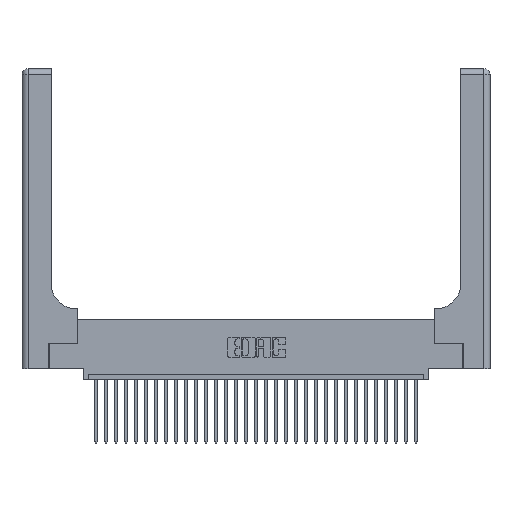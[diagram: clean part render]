
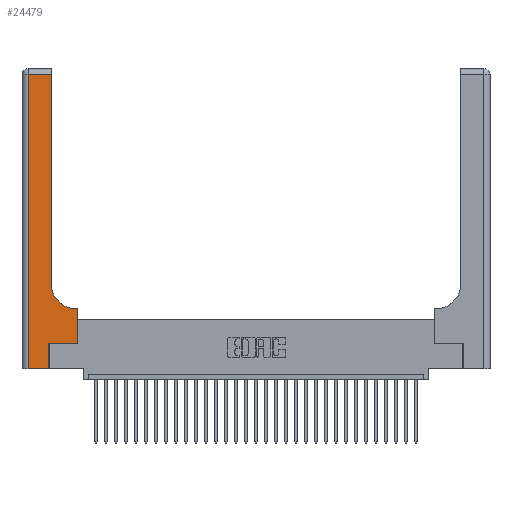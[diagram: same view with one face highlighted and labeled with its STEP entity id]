
A CAD part, top view. The second image highlights one B-rep face of the part: STEP entity #24479.
In plain terms, the highlighted planar face has unit normal (0, 0, 1).
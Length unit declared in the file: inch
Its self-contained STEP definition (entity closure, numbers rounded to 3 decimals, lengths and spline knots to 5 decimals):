
#134 = DIRECTION ( 'NONE',  ( 1., 0., 0. ) ) ;
#626 = VERTEX_POINT ( 'NONE', #4898 ) ;
#785 = DIRECTION ( 'NONE',  ( -1., 0., 0. ) ) ;
#903 = CARTESIAN_POINT ( 'NONE',  ( 0.2915, 0.85, 0.37 ) ) ;
#919 = CARTESIAN_POINT ( 'NONE',  ( 0.06, 3., 0.37 ) ) ;
#1185 = ORIENTED_EDGE ( 'NONE', *, *, #11596, .T. ) ;
#2694 = VERTEX_POINT ( 'NONE', #7220 ) ;
#2824 = VECTOR ( 'NONE', #3640, 39.37008 ) ;
#3193 = AXIS2_PLACEMENT_3D ( 'NONE', #12048, #14713, #22135 ) ;
#3640 = DIRECTION ( 'NONE',  ( 1., 0., 0. ) ) ;
#4898 = CARTESIAN_POINT ( 'NONE',  ( 0.5415, 0.6, 0.37 ) ) ;
#5334 = VECTOR ( 'NONE', #9507, 39.37008 ) ;
#6000 = EDGE_CURVE ( 'NONE', #26856, #626, #19930, .T. ) ;
#6341 = AXIS2_PLACEMENT_3D ( 'NONE', #24748, #12202, #134 ) ;
#7001 = EDGE_CURVE ( 'NONE', #15979, #7440, #29342, .T. ) ;
#7220 = CARTESIAN_POINT ( 'NONE',  ( 0.06, 2.94, 0.37 ) ) ;
#7440 = VERTEX_POINT ( 'NONE', #28754 ) ;
#8438 = CARTESIAN_POINT ( 'NONE',  ( 0.269, 0., 0.37 ) ) ;
#8507 = ORIENTED_EDGE ( 'NONE', *, *, #7001, .T. ) ;
#9351 = ORIENTED_EDGE ( 'NONE', *, *, #22669, .T. ) ;
#9507 = DIRECTION ( 'NONE',  ( 0., 1., 0. ) ) ;
#9606 = DIRECTION ( 'NONE',  ( -1., 0., 0. ) ) ;
#11596 = EDGE_CURVE ( 'NONE', #17450, #24165, #13840, .T. ) ;
#11725 = LINE ( 'NONE', #21700, #5334 ) ;
#12048 = CARTESIAN_POINT ( 'NONE',  ( 0., 3., 0.37 ) ) ;
#12202 = DIRECTION ( 'NONE',  ( 0., 0., -1. ) ) ;
#12247 = LINE ( 'NONE', #8438, #25920 ) ;
#13160 = ORIENTED_EDGE ( 'NONE', *, *, #29422, .T. ) ;
#13628 = EDGE_LOOP ( 'NONE', ( #19662, #9351, #13893, #1185, #20961, #8507, #16310, #20975, #13160 ) ) ;
#13840 = LINE ( 'NONE', #20938, #19926 ) ;
#13893 = ORIENTED_EDGE ( 'NONE', *, *, #29008, .T. ) ;
#14416 = CARTESIAN_POINT ( 'NONE',  ( 0.2915, 3., 0.37 ) ) ;
#14567 = EDGE_CURVE ( 'NONE', #24165, #15979, #12247, .T. ) ;
#14713 = DIRECTION ( 'NONE',  ( 0., 0., -1. ) ) ;
#15242 = DIRECTION ( 'NONE',  ( 0., 1., 0. ) ) ;
#15503 = EDGE_CURVE ( 'NONE', #21576, #30460, #17564, .T. ) ;
#15979 = VERTEX_POINT ( 'NONE', #17010 ) ;
#16278 = DIRECTION ( 'NONE',  ( 1., 0., 0. ) ) ;
#16310 = ORIENTED_EDGE ( 'NONE', *, *, #27569, .T. ) ;
#16707 = CARTESIAN_POINT ( 'NONE',  ( 0.2915, 0.6, 0.37 ) ) ;
#17010 = CARTESIAN_POINT ( 'NONE',  ( 0.269, 0.25, 0.37 ) ) ;
#17323 = CARTESIAN_POINT ( 'NONE',  ( 0.06, 0., 0.37 ) ) ;
#17450 = VERTEX_POINT ( 'NONE', #17323 ) ;
#17564 = LINE ( 'NONE', #14416, #17927 ) ;
#17927 = VECTOR ( 'NONE', #29030, 39.37008 ) ;
#17928 = CARTESIAN_POINT ( 'NONE',  ( 0.269, 0.25, 0.37 ) ) ;
#18076 = DIRECTION ( 'NONE',  ( 0., -1., 0. ) ) ;
#19619 = VECTOR ( 'NONE', #18076, 39.37008 ) ;
#19662 = ORIENTED_EDGE ( 'NONE', *, *, #15503, .T. ) ;
#19926 = VECTOR ( 'NONE', #16278, 39.37008 ) ;
#19930 = LINE ( 'NONE', #16707, #25617 ) ;
#20938 = CARTESIAN_POINT ( 'NONE',  ( 0., 0., 0.37 ) ) ;
#20961 = ORIENTED_EDGE ( 'NONE', *, *, #14567, .T. ) ;
#20975 = ORIENTED_EDGE ( 'NONE', *, *, #6000, .T. ) ;
#21080 = CARTESIAN_POINT ( 'NONE',  ( 0.2915, 2.94, 0.37 ) ) ;
#21526 = CARTESIAN_POINT ( 'NONE',  ( 0.269, 0., 0.37 ) ) ;
#21576 = VERTEX_POINT ( 'NONE', #903 ) ;
#21700 = CARTESIAN_POINT ( 'NONE',  ( 0.5585, 0.25, 0.37 ) ) ;
#22135 = DIRECTION ( 'NONE',  ( -1., 0., 0. ) ) ;
#22508 = CARTESIAN_POINT ( 'NONE',  ( 0., 2.94, 0.37 ) ) ;
#22669 = EDGE_CURVE ( 'NONE', #30460, #2694, #22686, .T. ) ;
#22686 = LINE ( 'NONE', #22508, #29107 ) ;
#23316 = FACE_OUTER_BOUND ( 'NONE', #13628, .T. ) ;
#24165 = VERTEX_POINT ( 'NONE', #21526 ) ;
#24479 = ADVANCED_FACE ( 'NONE', ( #23316 ), #27004, .F. ) ;
#24748 = CARTESIAN_POINT ( 'NONE',  ( 0.5415, 0.85, 0.37 ) ) ;
#25617 = VECTOR ( 'NONE', #9606, 39.37008 ) ;
#25920 = VECTOR ( 'NONE', #15242, 39.37008 ) ;
#26478 = CARTESIAN_POINT ( 'NONE',  ( 0.5585, 0.6, 0.37 ) ) ;
#26856 = VERTEX_POINT ( 'NONE', #26478 ) ;
#27004 = PLANE ( 'NONE',  #3193 ) ;
#27569 = EDGE_CURVE ( 'NONE', #7440, #26856, #11725, .T. ) ;
#28754 = CARTESIAN_POINT ( 'NONE',  ( 0.5585, 0.25, 0.37 ) ) ;
#29008 = EDGE_CURVE ( 'NONE', #2694, #17450, #30932, .T. ) ;
#29030 = DIRECTION ( 'NONE',  ( 0., 1., 0. ) ) ;
#29107 = VECTOR ( 'NONE', #785, 39.37008 ) ;
#29342 = LINE ( 'NONE', #17928, #2824 ) ;
#29422 = EDGE_CURVE ( 'NONE', #626, #21576, #30903, .T. ) ;
#30460 = VERTEX_POINT ( 'NONE', #21080 ) ;
#30903 = CIRCLE ( 'NONE', #6341, 0.25 ) ;
#30932 = LINE ( 'NONE', #919, #19619 ) ;
